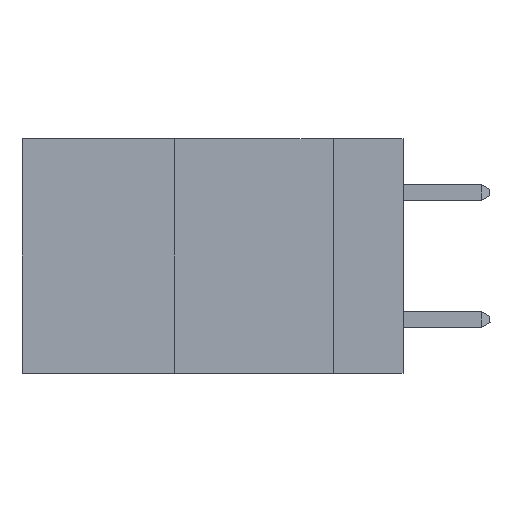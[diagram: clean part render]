
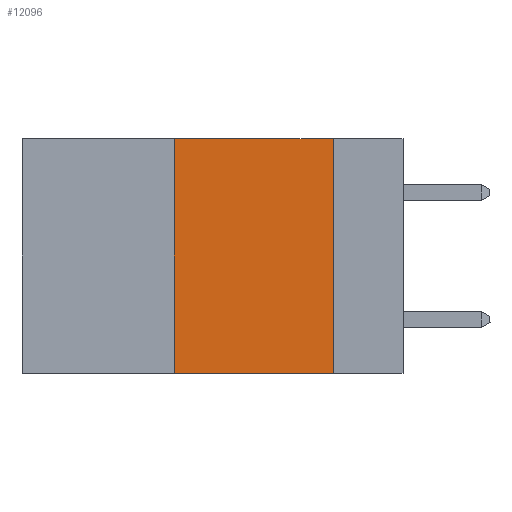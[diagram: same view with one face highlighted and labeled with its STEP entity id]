
A CAD part, left-side view. The second image highlights one B-rep face of the part: STEP entity #12096.
In plain terms, the highlighted planar face has unit normal (-1, 0, 0).
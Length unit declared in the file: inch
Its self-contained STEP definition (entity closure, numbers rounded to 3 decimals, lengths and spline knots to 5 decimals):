
#34 = CARTESIAN_POINT ( 'NONE',  ( 0., 0.11, 0. ) ) ;
#536 = ORIENTED_EDGE ( 'NONE', *, *, #12397, .T. ) ;
#694 = VECTOR ( 'NONE', #14034, 39.37008 ) ;
#1253 = DIRECTION ( 'NONE',  ( 0., 0., -1. ) ) ;
#1748 = CARTESIAN_POINT ( 'NONE',  ( 0., 0.6, 0. ) ) ;
#2413 = ORIENTED_EDGE ( 'NONE', *, *, #7311, .F. ) ;
#3794 = PLANE ( 'NONE',  #11151 ) ;
#3903 = CARTESIAN_POINT ( 'NONE',  ( 0., 0.11, 0. ) ) ;
#4071 = EDGE_CURVE ( 'NONE', #13328, #4959, #7610, .T. ) ;
#4959 = VERTEX_POINT ( 'NONE', #8526 ) ;
#5191 = CARTESIAN_POINT ( 'NONE',  ( 0., 0.6, -0.37 ) ) ;
#6284 = CARTESIAN_POINT ( 'NONE',  ( 0., 0.6, 0. ) ) ;
#6463 = LINE ( 'NONE', #5191, #9620 ) ;
#7213 = VECTOR ( 'NONE', #8983, 39.37008 ) ;
#7311 = EDGE_CURVE ( 'NONE', #8234, #14891, #14833, .T. ) ;
#7493 = DIRECTION ( 'NONE',  ( 0., 0., -1. ) ) ;
#7610 = LINE ( 'NONE', #14248, #694 ) ;
#8234 = VERTEX_POINT ( 'NONE', #3903 ) ;
#8236 = CARTESIAN_POINT ( 'NONE',  ( 0., 0.36, -0.37 ) ) ;
#8526 = CARTESIAN_POINT ( 'NONE',  ( 0., 0.36, 0. ) ) ;
#8983 = DIRECTION ( 'NONE',  ( 0., -1., 0. ) ) ;
#9515 = EDGE_CURVE ( 'NONE', #4959, #8234, #10018, .T. ) ;
#9620 = VECTOR ( 'NONE', #11201, 39.37008 ) ;
#10018 = LINE ( 'NONE', #1748, #7213 ) ;
#10342 = CARTESIAN_POINT ( 'NONE',  ( 0., 0.11, -0.37 ) ) ;
#10759 = ORIENTED_EDGE ( 'NONE', *, *, #4071, .F. ) ;
#11151 = AXIS2_PLACEMENT_3D ( 'NONE', #6284, #14525, #7493 ) ;
#11201 = DIRECTION ( 'NONE',  ( 0., -1., 0. ) ) ;
#11787 = VECTOR ( 'NONE', #1253, 39.37008 ) ;
#12096 = ADVANCED_FACE ( 'NONE', ( #13440 ), #3794, .F. ) ;
#12397 = EDGE_CURVE ( 'NONE', #13328, #14891, #6463, .T. ) ;
#12429 = ORIENTED_EDGE ( 'NONE', *, *, #9515, .F. ) ;
#13328 = VERTEX_POINT ( 'NONE', #8236 ) ;
#13440 = FACE_OUTER_BOUND ( 'NONE', #13714, .T. ) ;
#13714 = EDGE_LOOP ( 'NONE', ( #2413, #12429, #10759, #536 ) ) ;
#14034 = DIRECTION ( 'NONE',  ( 0., 0., 1. ) ) ;
#14248 = CARTESIAN_POINT ( 'NONE',  ( 0., 0.36, 0. ) ) ;
#14525 = DIRECTION ( 'NONE',  ( 1., 0., 0. ) ) ;
#14833 = LINE ( 'NONE', #34, #11787 ) ;
#14891 = VERTEX_POINT ( 'NONE', #10342 ) ;
